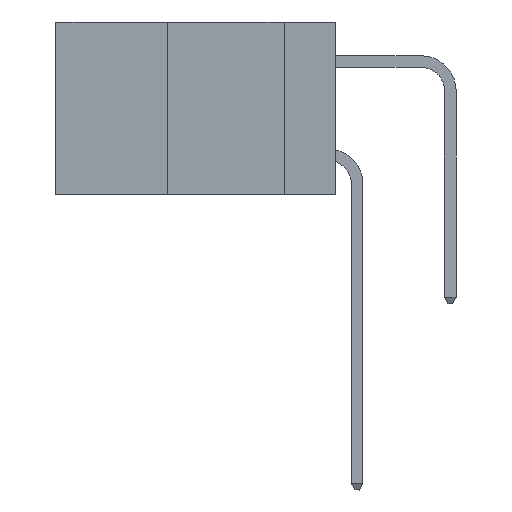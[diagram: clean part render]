
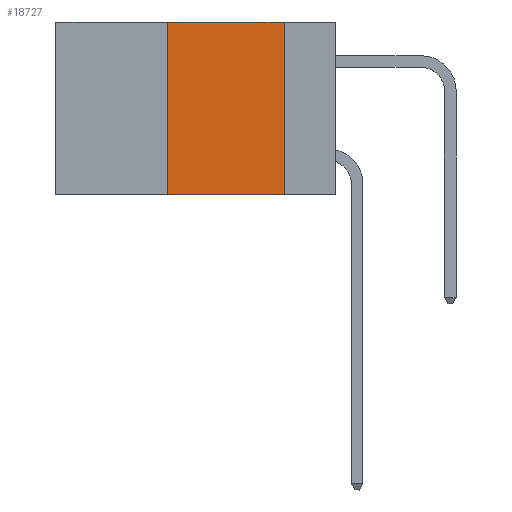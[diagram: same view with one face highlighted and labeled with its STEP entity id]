
A CAD part, left-side view. The second image highlights one B-rep face of the part: STEP entity #18727.
In plain terms, the highlighted planar face has unit normal (-1, 0, 0).
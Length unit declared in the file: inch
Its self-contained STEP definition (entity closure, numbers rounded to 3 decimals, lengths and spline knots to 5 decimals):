
#1331 = CARTESIAN_POINT ( 'NONE',  ( 0., 0.6, 0. ) ) ;
#1413 = VECTOR ( 'NONE', #13434, 39.37008 ) ;
#2914 = VECTOR ( 'NONE', #3811, 39.37008 ) ;
#2974 = AXIS2_PLACEMENT_3D ( 'NONE', #8705, #4398, #10244 ) ;
#3811 = DIRECTION ( 'NONE',  ( 0., 0., -1. ) ) ;
#4398 = DIRECTION ( 'NONE',  ( 1., 0., 0. ) ) ;
#4418 = CARTESIAN_POINT ( 'NONE',  ( 0., 0.36, 0. ) ) ;
#5083 = ORIENTED_EDGE ( 'NONE', *, *, #10049, .F. ) ;
#5394 = VERTEX_POINT ( 'NONE', #17317 ) ;
#5683 = CARTESIAN_POINT ( 'NONE',  ( 0., 0.6, -0.37 ) ) ;
#5987 = VERTEX_POINT ( 'NONE', #12102 ) ;
#6672 = EDGE_CURVE ( 'NONE', #12383, #8454, #13144, .T. ) ;
#7776 = ORIENTED_EDGE ( 'NONE', *, *, #12719, .T. ) ;
#8372 = LINE ( 'NONE', #5683, #9596 ) ;
#8454 = VERTEX_POINT ( 'NONE', #10246 ) ;
#8705 = CARTESIAN_POINT ( 'NONE',  ( 0., 0.6, 0. ) ) ;
#9219 = VECTOR ( 'NONE', #14074, 39.37008 ) ;
#9596 = VECTOR ( 'NONE', #15652, 39.37008 ) ;
#9843 = LINE ( 'NONE', #1331, #9219 ) ;
#9856 = CARTESIAN_POINT ( 'NONE',  ( 0., 0.36, -0.37 ) ) ;
#10049 = EDGE_CURVE ( 'NONE', #8454, #5394, #9843, .T. ) ;
#10244 = DIRECTION ( 'NONE',  ( 0., 0., -1. ) ) ;
#10246 = CARTESIAN_POINT ( 'NONE',  ( 0., 0.36, 0. ) ) ;
#11336 = EDGE_LOOP ( 'NONE', ( #13664, #5083, #15496, #7776 ) ) ;
#11500 = PLANE ( 'NONE',  #2974 ) ;
#12102 = CARTESIAN_POINT ( 'NONE',  ( 0., 0.11, -0.37 ) ) ;
#12383 = VERTEX_POINT ( 'NONE', #9856 ) ;
#12444 = CARTESIAN_POINT ( 'NONE',  ( 0., 0.11, 0. ) ) ;
#12719 = EDGE_CURVE ( 'NONE', #12383, #5987, #8372, .T. ) ;
#13144 = LINE ( 'NONE', #4418, #1413 ) ;
#13434 = DIRECTION ( 'NONE',  ( 0., 0., 1. ) ) ;
#13664 = ORIENTED_EDGE ( 'NONE', *, *, #16241, .F. ) ;
#14074 = DIRECTION ( 'NONE',  ( 0., -1., 0. ) ) ;
#14168 = LINE ( 'NONE', #12444, #2914 ) ;
#14661 = FACE_OUTER_BOUND ( 'NONE', #11336, .T. ) ;
#15496 = ORIENTED_EDGE ( 'NONE', *, *, #6672, .F. ) ;
#15652 = DIRECTION ( 'NONE',  ( 0., -1., 0. ) ) ;
#16241 = EDGE_CURVE ( 'NONE', #5394, #5987, #14168, .T. ) ;
#17317 = CARTESIAN_POINT ( 'NONE',  ( 0., 0.11, 0. ) ) ;
#18727 = ADVANCED_FACE ( 'NONE', ( #14661 ), #11500, .F. ) ;
